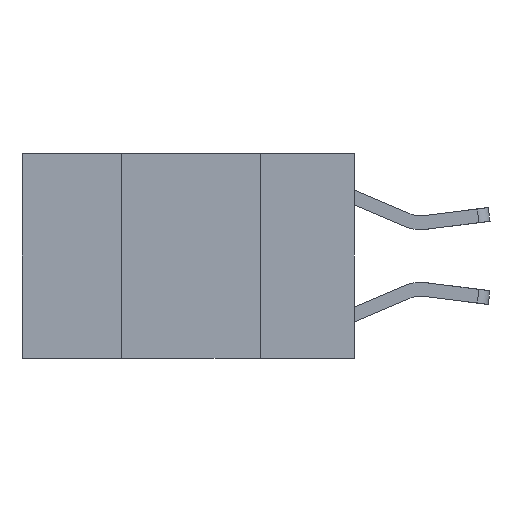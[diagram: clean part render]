
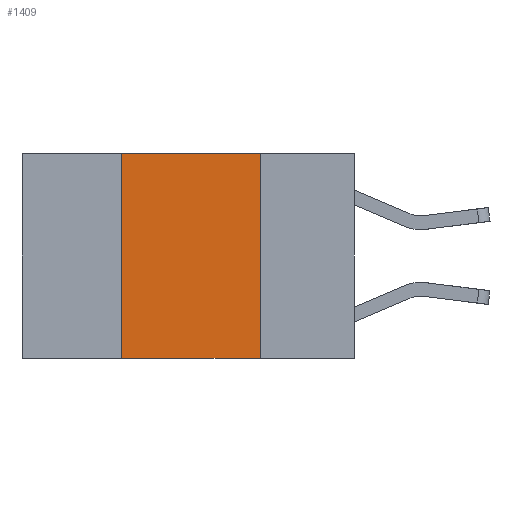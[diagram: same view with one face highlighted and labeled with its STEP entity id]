
A CAD part, left-side view. The second image highlights one B-rep face of the part: STEP entity #1409.
In plain terms, the highlighted planar face has unit normal (-1, 0, 0).
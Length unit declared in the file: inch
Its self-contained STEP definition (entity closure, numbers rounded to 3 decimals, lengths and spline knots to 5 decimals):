
#47 = CARTESIAN_POINT ( 'NONE',  ( 0., 0.17, 0. ) ) ;
#329 = CARTESIAN_POINT ( 'NONE',  ( 0., 0.17, 0. ) ) ;
#500 = CARTESIAN_POINT ( 'NONE',  ( 0., 0.6, -0.37 ) ) ;
#740 = VECTOR ( 'NONE', #9075, 39.37008 ) ;
#1131 = VECTOR ( 'NONE', #9217, 39.37008 ) ;
#1409 = ADVANCED_FACE ( 'NONE', ( #3838 ), #10108, .F. ) ;
#2200 = DIRECTION ( 'NONE',  ( 0., -1., 0. ) ) ;
#2219 = VERTEX_POINT ( 'NONE', #329 ) ;
#2522 = EDGE_LOOP ( 'NONE', ( #8400, #3692, #7871, #10457 ) ) ;
#2713 = DIRECTION ( 'NONE',  ( 1., 0., 0. ) ) ;
#3692 = ORIENTED_EDGE ( 'NONE', *, *, #5270, .F. ) ;
#3838 = FACE_OUTER_BOUND ( 'NONE', #2522, .T. ) ;
#3907 = LINE ( 'NONE', #500, #7995 ) ;
#3929 = VERTEX_POINT ( 'NONE', #5195 ) ;
#4242 = DIRECTION ( 'NONE',  ( 0., 0., -1. ) ) ;
#4245 = CARTESIAN_POINT ( 'NONE',  ( 0., 0.6, 0. ) ) ;
#4659 = EDGE_CURVE ( 'NONE', #3929, #5535, #7295, .T. ) ;
#5126 = CARTESIAN_POINT ( 'NONE',  ( 0., 0.6, 0. ) ) ;
#5195 = CARTESIAN_POINT ( 'NONE',  ( 0., 0.42, -0.37 ) ) ;
#5270 = EDGE_CURVE ( 'NONE', #5535, #2219, #5532, .T. ) ;
#5532 = LINE ( 'NONE', #4245, #1131 ) ;
#5535 = VERTEX_POINT ( 'NONE', #7846 ) ;
#6488 = VECTOR ( 'NONE', #4242, 39.37008 ) ;
#6810 = EDGE_CURVE ( 'NONE', #3929, #10035, #3907, .T. ) ;
#7182 = CARTESIAN_POINT ( 'NONE',  ( 0., 0.17, -0.37 ) ) ;
#7295 = LINE ( 'NONE', #8225, #740 ) ;
#7846 = CARTESIAN_POINT ( 'NONE',  ( 0., 0.42, 0. ) ) ;
#7871 = ORIENTED_EDGE ( 'NONE', *, *, #4659, .F. ) ;
#7995 = VECTOR ( 'NONE', #2200, 39.37008 ) ;
#8225 = CARTESIAN_POINT ( 'NONE',  ( 0., 0.42, 0. ) ) ;
#8400 = ORIENTED_EDGE ( 'NONE', *, *, #9430, .F. ) ;
#8424 = DIRECTION ( 'NONE',  ( 0., 0., -1. ) ) ;
#8723 = LINE ( 'NONE', #47, #6488 ) ;
#9075 = DIRECTION ( 'NONE',  ( 0., 0., 1. ) ) ;
#9217 = DIRECTION ( 'NONE',  ( 0., -1., 0. ) ) ;
#9430 = EDGE_CURVE ( 'NONE', #2219, #10035, #8723, .T. ) ;
#9530 = AXIS2_PLACEMENT_3D ( 'NONE', #5126, #2713, #8424 ) ;
#10035 = VERTEX_POINT ( 'NONE', #7182 ) ;
#10108 = PLANE ( 'NONE',  #9530 ) ;
#10457 = ORIENTED_EDGE ( 'NONE', *, *, #6810, .T. ) ;
